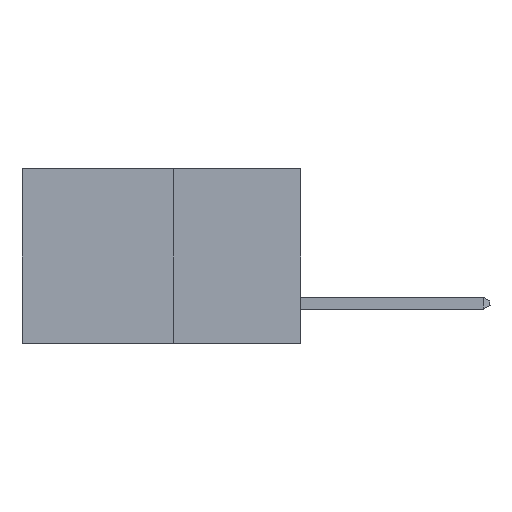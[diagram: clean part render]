
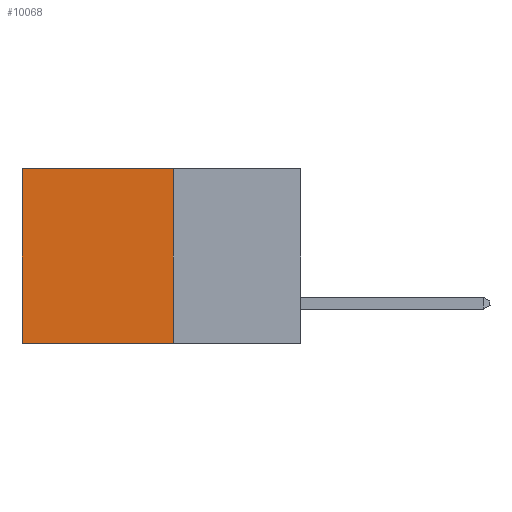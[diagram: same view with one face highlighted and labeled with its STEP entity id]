
A CAD part, left-side view. The second image highlights one B-rep face of the part: STEP entity #10068.
In plain terms, the highlighted planar face has unit normal (-1, 0, 0).
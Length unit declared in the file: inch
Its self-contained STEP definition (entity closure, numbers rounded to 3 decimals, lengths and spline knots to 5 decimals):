
#904 = CARTESIAN_POINT ( 'NONE',  ( 0.277, 0.27, 0. ) ) ;
#1525 = VERTEX_POINT ( 'NONE', #12469 ) ;
#2644 = LINE ( 'NONE', #8923, #5989 ) ;
#2694 = DIRECTION ( 'NONE',  ( 1., 0., 0. ) ) ;
#2720 = VERTEX_POINT ( 'NONE', #13427 ) ;
#2931 = CARTESIAN_POINT ( 'NONE',  ( 0.277, 0.59, 0. ) ) ;
#3105 = DIRECTION ( 'NONE',  ( 0., 0., -1. ) ) ;
#4077 = CARTESIAN_POINT ( 'NONE',  ( 0.277, 0.27, 0. ) ) ;
#5537 = DIRECTION ( 'NONE',  ( 0., 1., 0. ) ) ;
#5989 = VECTOR ( 'NONE', #3105, 39.37008 ) ;
#6915 = VECTOR ( 'NONE', #7633, 39.37008 ) ;
#7121 = LINE ( 'NONE', #9925, #10190 ) ;
#7229 = VERTEX_POINT ( 'NONE', #904 ) ;
#7374 = LINE ( 'NONE', #16499, #6915 ) ;
#7433 = EDGE_LOOP ( 'NONE', ( #15293, #13431, #15879, #15318 ) ) ;
#7633 = DIRECTION ( 'NONE',  ( 0., 0., -1. ) ) ;
#7859 = LINE ( 'NONE', #4077, #11422 ) ;
#8716 = FACE_OUTER_BOUND ( 'NONE', #7433, .T. ) ;
#8776 = EDGE_CURVE ( 'NONE', #1525, #2720, #7121, .T. ) ;
#8923 = CARTESIAN_POINT ( 'NONE',  ( 0.277, 0.27, -0.37 ) ) ;
#9467 = AXIS2_PLACEMENT_3D ( 'NONE', #15834, #2694, #12991 ) ;
#9925 = CARTESIAN_POINT ( 'NONE',  ( 0.277, 0.27, -0.37 ) ) ;
#10068 = ADVANCED_FACE ( 'NONE', ( #8716 ), #17253, .F. ) ;
#10190 = VECTOR ( 'NONE', #18580, 39.37008 ) ;
#11422 = VECTOR ( 'NONE', #5537, 39.37008 ) ;
#12469 = CARTESIAN_POINT ( 'NONE',  ( 0.277, 0.27, -0.37 ) ) ;
#12991 = DIRECTION ( 'NONE',  ( 0., 0., -1. ) ) ;
#13427 = CARTESIAN_POINT ( 'NONE',  ( 0.277, 0.59, -0.37 ) ) ;
#13431 = ORIENTED_EDGE ( 'NONE', *, *, #8776, .F. ) ;
#14232 = VERTEX_POINT ( 'NONE', #2931 ) ;
#14660 = EDGE_CURVE ( 'NONE', #7229, #14232, #7859, .T. ) ;
#15293 = ORIENTED_EDGE ( 'NONE', *, *, #16318, .T. ) ;
#15318 = ORIENTED_EDGE ( 'NONE', *, *, #14660, .T. ) ;
#15834 = CARTESIAN_POINT ( 'NONE',  ( 0.277, 0.27, -0.37 ) ) ;
#15879 = ORIENTED_EDGE ( 'NONE', *, *, #16765, .F. ) ;
#16318 = EDGE_CURVE ( 'NONE', #14232, #2720, #7374, .T. ) ;
#16499 = CARTESIAN_POINT ( 'NONE',  ( 0.277, 0.59, -0.37 ) ) ;
#16765 = EDGE_CURVE ( 'NONE', #7229, #1525, #2644, .T. ) ;
#17253 = PLANE ( 'NONE',  #9467 ) ;
#18580 = DIRECTION ( 'NONE',  ( 0., 1., 0. ) ) ;
